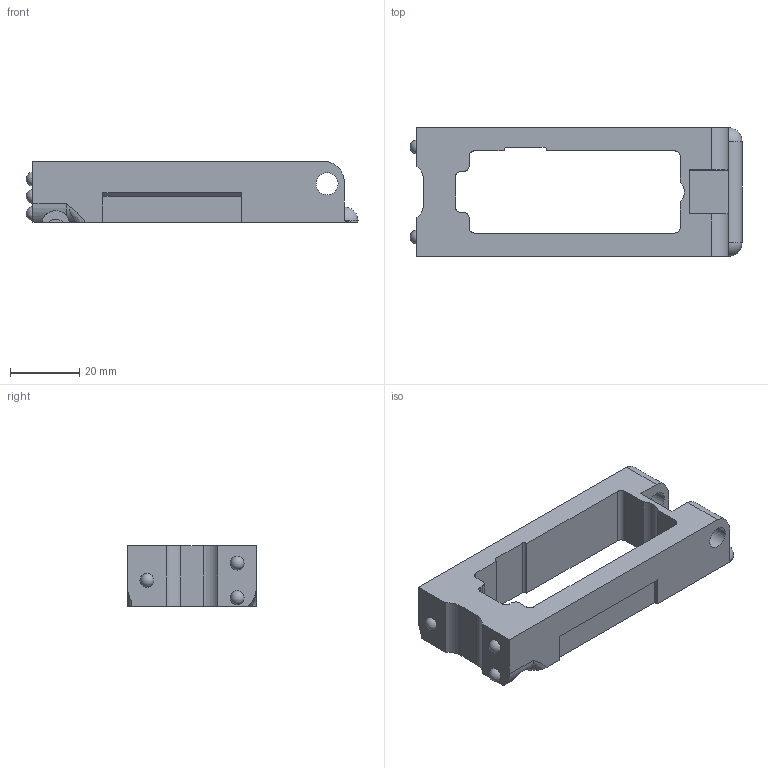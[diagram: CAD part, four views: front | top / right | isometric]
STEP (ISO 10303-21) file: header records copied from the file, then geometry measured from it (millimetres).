
FILE_DESCRIPTION (( 'STEP AP214' ), '1' );
FILE_NAME ('Magwell_1.STEP', '2015-10-23T19:50:15', ( 'WarFairy' ), ( '' ), 'SwSTEP 2.0', 'SolidWorks 2015', '' );
FILE_SCHEMA (( 'AUTOMOTIVE_DESIGN' ));
Length unit declared in the file: millimetre
Products named in the file (1): Magwell_1
Bounding box: 95.81 x 37.13 x 17.46 mm (x, y, z)
Volume: 28280.6 mm3; surface area: 12144.9 mm2
Topology: 1 solids, 2 shells, 91 faces, 273 edges, 182 vertices
Faces by surface type: plane 41, cylinder 30, sphere 18, bspline 1, torus 1
Entity records: 2998 total; most frequent: CARTESIAN_POINT 621, DIRECTION 496, ORIENTED_EDGE 476, EDGE_CURVE 238, AXIS2_PLACEMENT_3D 180, VERTEX_POINT 165, LINE 136, VECTOR 136
